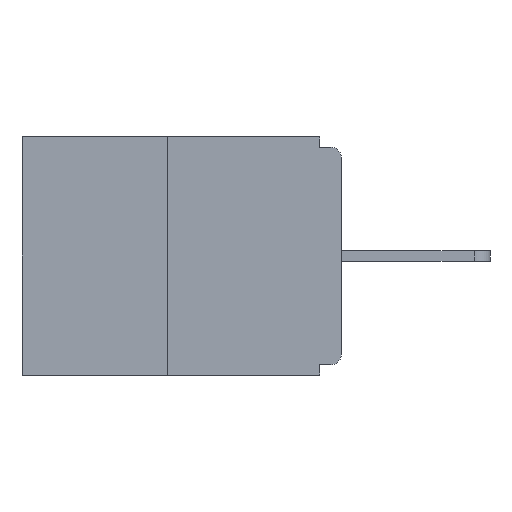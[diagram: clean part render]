
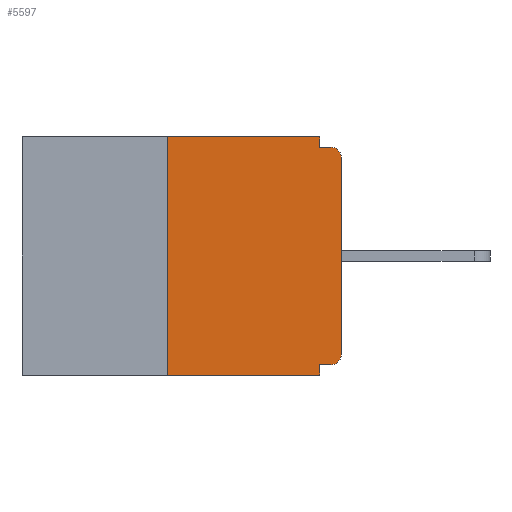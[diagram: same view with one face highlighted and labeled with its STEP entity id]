
A CAD part, left-side view. The second image highlights one B-rep face of the part: STEP entity #5597.
In plain terms, the highlighted planar face has unit normal (-1, 0, 0).
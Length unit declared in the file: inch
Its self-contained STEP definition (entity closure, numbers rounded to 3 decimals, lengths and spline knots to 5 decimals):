
#1 = DIRECTION ( 'NONE',  ( 0., 0., 1. ) ) ;
#205 = LINE ( 'NONE', #982, #6618 ) ;
#263 = VERTEX_POINT ( 'NONE', #6205 ) ;
#312 = VECTOR ( 'NONE', #11291, 39.37008 ) ;
#584 = EDGE_CURVE ( 'NONE', #7905, #6722, #7389, .T. ) ;
#706 = VECTOR ( 'NONE', #8916, 39.37008 ) ;
#901 = DIRECTION ( 'NONE',  ( 0., 0., -1. ) ) ;
#919 = EDGE_CURVE ( 'NONE', #7905, #7735, #8515, .T. ) ;
#982 = CARTESIAN_POINT ( 'NONE',  ( 0., 0.031, -0.343 ) ) ;
#1426 = ORIENTED_EDGE ( 'NONE', *, *, #4648, .F. ) ;
#1445 = ORIENTED_EDGE ( 'NONE', *, *, #584, .F. ) ;
#1579 = CARTESIAN_POINT ( 'NONE',  ( 0., 0.46, 0. ) ) ;
#1606 = ORIENTED_EDGE ( 'NONE', *, *, #919, .T. ) ;
#1646 = ORIENTED_EDGE ( 'NONE', *, *, #6366, .F. ) ;
#1654 = FACE_OUTER_BOUND ( 'NONE', #5510, .T. ) ;
#1758 = DIRECTION ( 'NONE',  ( 0., 0., -1. ) ) ;
#1770 = ORIENTED_EDGE ( 'NONE', *, *, #7670, .F. ) ;
#1773 = ORIENTED_EDGE ( 'NONE', *, *, #10982, .T. ) ;
#1815 = CARTESIAN_POINT ( 'NONE',  ( 0., 0.031, 0. ) ) ;
#1884 = ORIENTED_EDGE ( 'NONE', *, *, #9337, .T. ) ;
#1900 = ORIENTED_EDGE ( 'NONE', *, *, #12186, .T. ) ;
#2032 = ORIENTED_EDGE ( 'NONE', *, *, #10131, .F. ) ;
#2043 = ORIENTED_EDGE ( 'NONE', *, *, #9652, .F. ) ;
#2559 = DIRECTION ( 'NONE',  ( 0., 0., -1. ) ) ;
#2583 = DIRECTION ( 'NONE',  ( -1., 0., 0. ) ) ;
#2605 = CARTESIAN_POINT ( 'NONE',  ( 0., 0.015, -0.313 ) ) ;
#3297 = CIRCLE ( 'NONE', #12868, 0.015 ) ;
#3322 = VERTEX_POINT ( 'NONE', #11598 ) ;
#3970 = CARTESIAN_POINT ( 'NONE',  ( 0., 0.46, -0.343 ) ) ;
#3984 = DIRECTION ( 'NONE',  ( 0., -1., 0. ) ) ;
#4107 = LINE ( 'NONE', #11652, #10564 ) ;
#4209 = LINE ( 'NONE', #10065, #13539 ) ;
#4648 = EDGE_CURVE ( 'NONE', #6722, #5851, #7471, .T. ) ;
#5012 = CARTESIAN_POINT ( 'NONE',  ( 0., 0.015, -0.328 ) ) ;
#5053 = CARTESIAN_POINT ( 'NONE',  ( 0., 0.031, -0.015 ) ) ;
#5200 = VECTOR ( 'NONE', #3984, 39.37008 ) ;
#5510 = EDGE_LOOP ( 'NONE', ( #1426, #1445, #1606, #1646, #1770, #1773, #1884, #1900, #2032, #2043 ) ) ;
#5597 = ADVANCED_FACE ( 'NONE', ( #1654 ), #7479, .F. ) ;
#5851 = VERTEX_POINT ( 'NONE', #12571 ) ;
#6205 = CARTESIAN_POINT ( 'NONE',  ( 0., 0.015, -0.015 ) ) ;
#6366 = EDGE_CURVE ( 'NONE', #6793, #7735, #205, .T. ) ;
#6618 = VECTOR ( 'NONE', #901, 39.37008 ) ;
#6722 = VERTEX_POINT ( 'NONE', #15648 ) ;
#6793 = VERTEX_POINT ( 'NONE', #11466 ) ;
#6797 = CARTESIAN_POINT ( 'NONE',  ( 0., 0.46, 0. ) ) ;
#7104 = LINE ( 'NONE', #13322, #312 ) ;
#7389 = LINE ( 'NONE', #13543, #12959 ) ;
#7471 = LINE ( 'NONE', #1579, #706 ) ;
#7479 = PLANE ( 'NONE',  #8888 ) ;
#7670 = EDGE_CURVE ( 'NONE', #11850, #6793, #4209, .T. ) ;
#7735 = VERTEX_POINT ( 'NONE', #8005 ) ;
#7905 = VERTEX_POINT ( 'NONE', #12672 ) ;
#8005 = CARTESIAN_POINT ( 'NONE',  ( 0., 0.031, -0.343 ) ) ;
#8075 = DIRECTION ( 'NONE',  ( 1., 0., 0. ) ) ;
#8113 = DIRECTION ( 'NONE',  ( 0., 0., -1. ) ) ;
#8263 = VECTOR ( 'NONE', #1758, 39.37008 ) ;
#8515 = LINE ( 'NONE', #3970, #5200 ) ;
#8888 = AXIS2_PLACEMENT_3D ( 'NONE', #6797, #8075, #8113 ) ;
#8916 = DIRECTION ( 'NONE',  ( 0., -1., 0. ) ) ;
#9115 = CARTESIAN_POINT ( 'NONE',  ( 0., 0., -0.313 ) ) ;
#9151 = CIRCLE ( 'NONE', #11374, 0.015 ) ;
#9337 = EDGE_CURVE ( 'NONE', #11615, #3322, #7104, .T. ) ;
#9652 = EDGE_CURVE ( 'NONE', #5851, #15415, #14549, .T. ) ;
#10065 = CARTESIAN_POINT ( 'NONE',  ( 0., 0., -0.328 ) ) ;
#10131 = EDGE_CURVE ( 'NONE', #15415, #263, #4107, .T. ) ;
#10564 = VECTOR ( 'NONE', #11816, 39.37008 ) ;
#10982 = EDGE_CURVE ( 'NONE', #11850, #11615, #9151, .T. ) ;
#11291 = DIRECTION ( 'NONE',  ( 0., 0., 1. ) ) ;
#11350 = DIRECTION ( 'NONE',  ( 0., 1., 0. ) ) ;
#11374 = AXIS2_PLACEMENT_3D ( 'NONE', #2605, #2583, #2559 ) ;
#11466 = CARTESIAN_POINT ( 'NONE',  ( 0., 0.031, -0.328 ) ) ;
#11598 = CARTESIAN_POINT ( 'NONE',  ( 0., 0., -0.03 ) ) ;
#11615 = VERTEX_POINT ( 'NONE', #9115 ) ;
#11652 = CARTESIAN_POINT ( 'NONE',  ( 0., 0., -0.015 ) ) ;
#11816 = DIRECTION ( 'NONE',  ( 0., -1., 0. ) ) ;
#11850 = VERTEX_POINT ( 'NONE', #5012 ) ;
#12186 = EDGE_CURVE ( 'NONE', #3322, #263, #3297, .T. ) ;
#12571 = CARTESIAN_POINT ( 'NONE',  ( 0., 0.031, 0. ) ) ;
#12672 = CARTESIAN_POINT ( 'NONE',  ( 0., 0.25, -0.343 ) ) ;
#12868 = AXIS2_PLACEMENT_3D ( 'NONE', #14775, #14753, #14730 ) ;
#12959 = VECTOR ( 'NONE', #1, 39.37008 ) ;
#13322 = CARTESIAN_POINT ( 'NONE',  ( 0., 0., 0. ) ) ;
#13539 = VECTOR ( 'NONE', #11350, 39.37008 ) ;
#13543 = CARTESIAN_POINT ( 'NONE',  ( 0., 0.25, 0. ) ) ;
#14549 = LINE ( 'NONE', #1815, #8263 ) ;
#14730 = DIRECTION ( 'NONE',  ( 0., 0., -1. ) ) ;
#14753 = DIRECTION ( 'NONE',  ( -1., 0., 0. ) ) ;
#14775 = CARTESIAN_POINT ( 'NONE',  ( 0., 0.015, -0.03 ) ) ;
#15415 = VERTEX_POINT ( 'NONE', #5053 ) ;
#15648 = CARTESIAN_POINT ( 'NONE',  ( 0., 0.25, 0. ) ) ;
